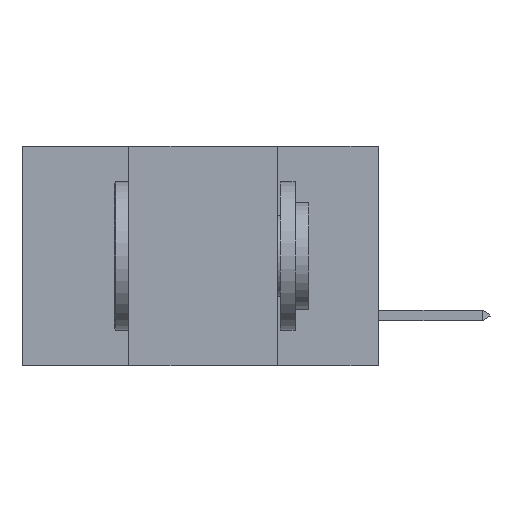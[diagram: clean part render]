
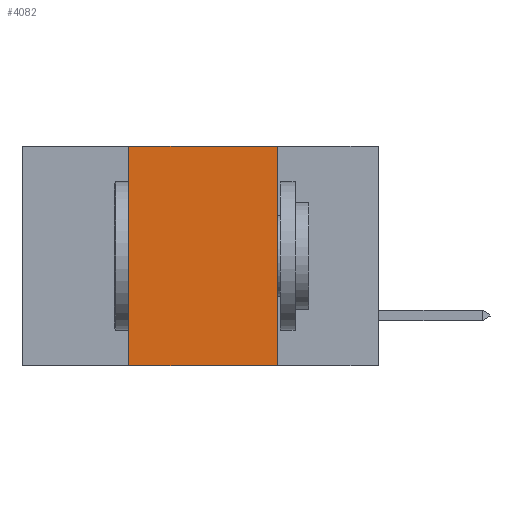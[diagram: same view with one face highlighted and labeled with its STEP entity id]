
A CAD part, left-side view. The second image highlights one B-rep face of the part: STEP entity #4082.
In plain terms, the highlighted planar face has unit normal (-1, 0, 0).
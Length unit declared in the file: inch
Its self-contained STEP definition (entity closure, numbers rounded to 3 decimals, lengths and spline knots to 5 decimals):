
#573 = EDGE_LOOP ( 'NONE', ( #2007, #7972, #7365, #5224 ) ) ;
#601 = EDGE_CURVE ( 'NONE', #9199, #5092, #12526, .T. ) ;
#878 = VECTOR ( 'NONE', #12350, 39.37008 ) ;
#1304 = VECTOR ( 'NONE', #3678, 39.37008 ) ;
#1516 = CARTESIAN_POINT ( 'NONE',  ( 0., 0.42, 0. ) ) ;
#1568 = DIRECTION ( 'NONE',  ( 0., 0., 1. ) ) ;
#1573 = CARTESIAN_POINT ( 'NONE',  ( 0., 0.17, 0. ) ) ;
#1720 = FACE_OUTER_BOUND ( 'NONE', #573, .T. ) ;
#2007 = ORIENTED_EDGE ( 'NONE', *, *, #4246, .F. ) ;
#3678 = DIRECTION ( 'NONE',  ( 0., -1., 0. ) ) ;
#3923 = DIRECTION ( 'NONE',  ( 0., 0., -1. ) ) ;
#4032 = CARTESIAN_POINT ( 'NONE',  ( 0., 0.6, -0.37 ) ) ;
#4082 = ADVANCED_FACE ( 'NONE', ( #1720 ), #9396, .F. ) ;
#4246 = EDGE_CURVE ( 'NONE', #9601, #13140, #14685, .T. ) ;
#4933 = DIRECTION ( 'NONE',  ( 0., 0., -1. ) ) ;
#5092 = VERTEX_POINT ( 'NONE', #6790 ) ;
#5224 = ORIENTED_EDGE ( 'NONE', *, *, #10936, .T. ) ;
#6767 = CARTESIAN_POINT ( 'NONE',  ( 0., 0.17, -0.37 ) ) ;
#6790 = CARTESIAN_POINT ( 'NONE',  ( 0., 0.42, 0. ) ) ;
#7007 = LINE ( 'NONE', #11207, #878 ) ;
#7365 = ORIENTED_EDGE ( 'NONE', *, *, #601, .F. ) ;
#7431 = LINE ( 'NONE', #4032, #1304 ) ;
#7972 = ORIENTED_EDGE ( 'NONE', *, *, #12261, .F. ) ;
#9199 = VERTEX_POINT ( 'NONE', #14171 ) ;
#9396 = PLANE ( 'NONE',  #12704 ) ;
#9469 = VECTOR ( 'NONE', #3923, 39.37008 ) ;
#9601 = VERTEX_POINT ( 'NONE', #14584 ) ;
#10695 = DIRECTION ( 'NONE',  ( 1., 0., 0. ) ) ;
#10936 = EDGE_CURVE ( 'NONE', #9199, #13140, #7431, .T. ) ;
#11207 = CARTESIAN_POINT ( 'NONE',  ( 0., 0.6, 0. ) ) ;
#11299 = VECTOR ( 'NONE', #1568, 39.37008 ) ;
#12261 = EDGE_CURVE ( 'NONE', #5092, #9601, #7007, .T. ) ;
#12350 = DIRECTION ( 'NONE',  ( 0., -1., 0. ) ) ;
#12526 = LINE ( 'NONE', #1516, #11299 ) ;
#12704 = AXIS2_PLACEMENT_3D ( 'NONE', #12855, #10695, #4933 ) ;
#12855 = CARTESIAN_POINT ( 'NONE',  ( 0., 0.6, 0. ) ) ;
#13140 = VERTEX_POINT ( 'NONE', #6767 ) ;
#14171 = CARTESIAN_POINT ( 'NONE',  ( 0., 0.42, -0.37 ) ) ;
#14584 = CARTESIAN_POINT ( 'NONE',  ( 0., 0.17, 0. ) ) ;
#14685 = LINE ( 'NONE', #1573, #9469 ) ;
